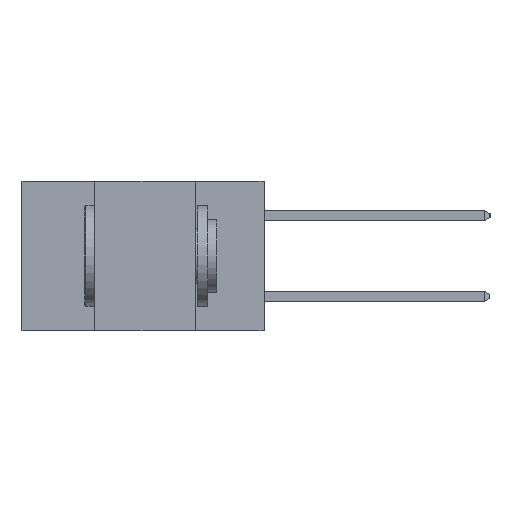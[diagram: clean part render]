
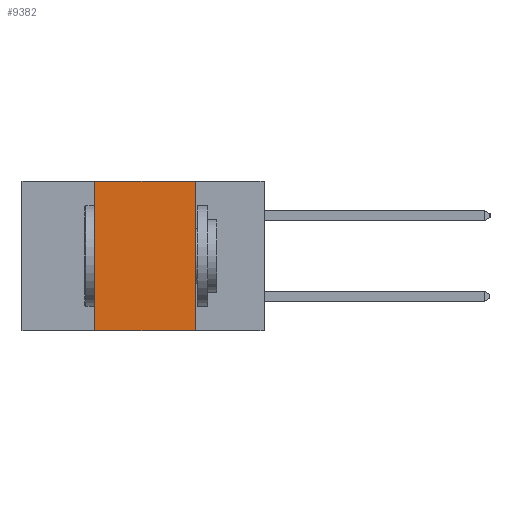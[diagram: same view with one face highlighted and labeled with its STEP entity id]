
A CAD part, left-side view. The second image highlights one B-rep face of the part: STEP entity #9382.
In plain terms, the highlighted planar face has unit normal (-1, 0, 0).
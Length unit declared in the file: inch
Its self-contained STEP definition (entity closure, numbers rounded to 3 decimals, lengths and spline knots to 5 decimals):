
#314 = DIRECTION ( 'NONE',  ( 0., 0., -1. ) ) ;
#748 = CARTESIAN_POINT ( 'NONE',  ( 0., 0.6, 0. ) ) ;
#1353 = LINE ( 'NONE', #11837, #3502 ) ;
#1539 = CARTESIAN_POINT ( 'NONE',  ( 0., 0.17, -0.37 ) ) ;
#1572 = ORIENTED_EDGE ( 'NONE', *, *, #10548, .T. ) ;
#1903 = DIRECTION ( 'NONE',  ( 0., 0., -1. ) ) ;
#2157 = VECTOR ( 'NONE', #12833, 39.37008 ) ;
#2400 = DIRECTION ( 'NONE',  ( 0., -1., 0. ) ) ;
#2813 = AXIS2_PLACEMENT_3D ( 'NONE', #748, #12269, #1903 ) ;
#2882 = CARTESIAN_POINT ( 'NONE',  ( 0., 0.17, -0.37 ) ) ;
#3222 = CARTESIAN_POINT ( 'NONE',  ( 0., 0.42, -0.37 ) ) ;
#3502 = VECTOR ( 'NONE', #4334, 39.37008 ) ;
#3799 = ORIENTED_EDGE ( 'NONE', *, *, #8233, .F. ) ;
#4193 = VERTEX_POINT ( 'NONE', #2882 ) ;
#4302 = CARTESIAN_POINT ( 'NONE',  ( 0., 0.42, -0.37 ) ) ;
#4334 = DIRECTION ( 'NONE',  ( 0., -1., 0. ) ) ;
#5610 = LINE ( 'NONE', #4302, #2157 ) ;
#5656 = ORIENTED_EDGE ( 'NONE', *, *, #12774, .F. ) ;
#5775 = VECTOR ( 'NONE', #314, 39.37008 ) ;
#5931 = VERTEX_POINT ( 'NONE', #13230 ) ;
#6004 = FACE_OUTER_BOUND ( 'NONE', #13224, .T. ) ;
#6867 = VERTEX_POINT ( 'NONE', #8159 ) ;
#7579 = LINE ( 'NONE', #11729, #12161 ) ;
#8159 = CARTESIAN_POINT ( 'NONE',  ( 0., 0.42, 0. ) ) ;
#8173 = PLANE ( 'NONE',  #2813 ) ;
#8233 = EDGE_CURVE ( 'NONE', #5931, #4193, #10814, .T. ) ;
#9382 = ADVANCED_FACE ( 'NONE', ( #6004 ), #8173, .F. ) ;
#10548 = EDGE_CURVE ( 'NONE', #12234, #4193, #7579, .T. ) ;
#10814 = LINE ( 'NONE', #1539, #5775 ) ;
#11463 = ORIENTED_EDGE ( 'NONE', *, *, #12032, .F. ) ;
#11729 = CARTESIAN_POINT ( 'NONE',  ( 0., 0.6, -0.37 ) ) ;
#11837 = CARTESIAN_POINT ( 'NONE',  ( 0., 0.6, 0. ) ) ;
#12032 = EDGE_CURVE ( 'NONE', #12234, #6867, #5610, .T. ) ;
#12161 = VECTOR ( 'NONE', #2400, 39.37008 ) ;
#12234 = VERTEX_POINT ( 'NONE', #3222 ) ;
#12269 = DIRECTION ( 'NONE',  ( 1., 0., 0. ) ) ;
#12774 = EDGE_CURVE ( 'NONE', #6867, #5931, #1353, .T. ) ;
#12833 = DIRECTION ( 'NONE',  ( 0., 0., 1. ) ) ;
#13224 = EDGE_LOOP ( 'NONE', ( #3799, #5656, #11463, #1572 ) ) ;
#13230 = CARTESIAN_POINT ( 'NONE',  ( 0., 0.17, 0. ) ) ;
